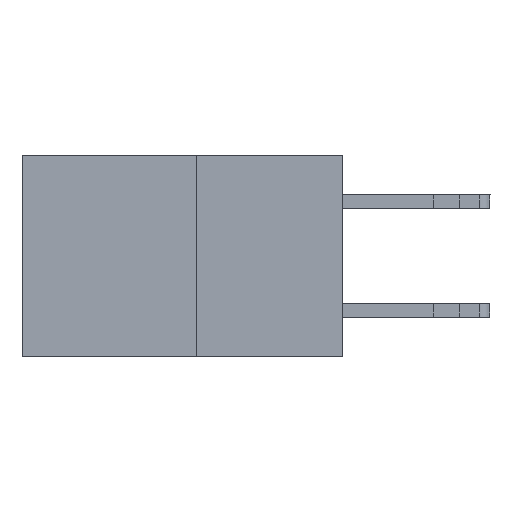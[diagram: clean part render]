
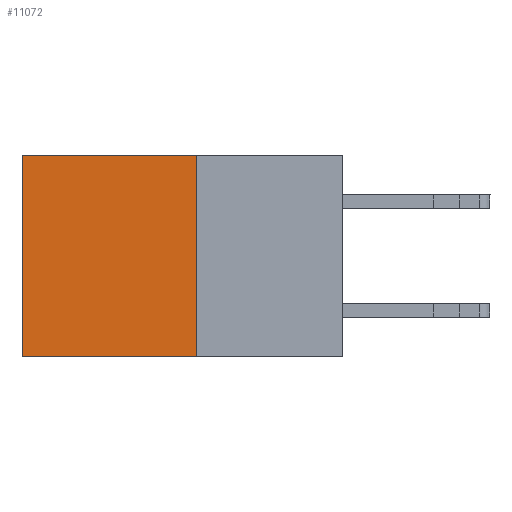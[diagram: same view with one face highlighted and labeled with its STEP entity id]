
A CAD part, left-side view. The second image highlights one B-rep face of the part: STEP entity #11072.
In plain terms, the highlighted planar face has unit normal (-1, 0, 0).
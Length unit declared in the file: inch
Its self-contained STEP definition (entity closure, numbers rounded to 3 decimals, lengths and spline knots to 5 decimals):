
#568 = EDGE_LOOP ( 'NONE', ( #12372, #11966, #10330, #10537 ) ) ;
#2612 = FACE_OUTER_BOUND ( 'NONE', #568, .T. ) ;
#2632 = CARTESIAN_POINT ( 'NONE',  ( 0.277, 0.27, -0.37 ) ) ;
#2668 = CARTESIAN_POINT ( 'NONE',  ( 0.277, 0.59, 0. ) ) ;
#2954 = VECTOR ( 'NONE', #13649, 39.37008 ) ;
#3480 = VECTOR ( 'NONE', #8361, 39.37008 ) ;
#4029 = DIRECTION ( 'NONE',  ( 0., 0., -1. ) ) ;
#4634 = EDGE_CURVE ( 'NONE', #5257, #15566, #16468, .T. ) ;
#4862 = CARTESIAN_POINT ( 'NONE',  ( 0.277, 0.27, 0. ) ) ;
#5257 = VERTEX_POINT ( 'NONE', #14742 ) ;
#6990 = CARTESIAN_POINT ( 'NONE',  ( 0.277, 0.27, -0.37 ) ) ;
#7020 = LINE ( 'NONE', #7182, #3480 ) ;
#7182 = CARTESIAN_POINT ( 'NONE',  ( 0.277, 0.59, -0.37 ) ) ;
#7238 = CARTESIAN_POINT ( 'NONE',  ( 0.277, 0.59, -0.37 ) ) ;
#8361 = DIRECTION ( 'NONE',  ( 0., 0., -1. ) ) ;
#8503 = LINE ( 'NONE', #6990, #2954 ) ;
#10330 = ORIENTED_EDGE ( 'NONE', *, *, #10469, .F. ) ;
#10469 = EDGE_CURVE ( 'NONE', #5257, #13905, #11695, .T. ) ;
#10500 = PLANE ( 'NONE',  #13161 ) ;
#10537 = ORIENTED_EDGE ( 'NONE', *, *, #4634, .T. ) ;
#10772 = VECTOR ( 'NONE', #15183, 39.37008 ) ;
#11072 = ADVANCED_FACE ( 'NONE', ( #2612 ), #10500, .F. ) ;
#11477 = CARTESIAN_POINT ( 'NONE',  ( 0.277, 0.27, -0.37 ) ) ;
#11613 = DIRECTION ( 'NONE',  ( 0., 0., -1. ) ) ;
#11695 = LINE ( 'NONE', #2632, #12873 ) ;
#11966 = ORIENTED_EDGE ( 'NONE', *, *, #14283, .F. ) ;
#12372 = ORIENTED_EDGE ( 'NONE', *, *, #15162, .T. ) ;
#12873 = VECTOR ( 'NONE', #11613, 39.37008 ) ;
#13161 = AXIS2_PLACEMENT_3D ( 'NONE', #15636, #16669, #4029 ) ;
#13649 = DIRECTION ( 'NONE',  ( 0., 1., 0. ) ) ;
#13905 = VERTEX_POINT ( 'NONE', #11477 ) ;
#14249 = VERTEX_POINT ( 'NONE', #7238 ) ;
#14283 = EDGE_CURVE ( 'NONE', #13905, #14249, #8503, .T. ) ;
#14742 = CARTESIAN_POINT ( 'NONE',  ( 0.277, 0.27, 0. ) ) ;
#15162 = EDGE_CURVE ( 'NONE', #15566, #14249, #7020, .T. ) ;
#15183 = DIRECTION ( 'NONE',  ( 0., 1., 0. ) ) ;
#15566 = VERTEX_POINT ( 'NONE', #2668 ) ;
#15636 = CARTESIAN_POINT ( 'NONE',  ( 0.277, 0.27, -0.37 ) ) ;
#16468 = LINE ( 'NONE', #4862, #10772 ) ;
#16669 = DIRECTION ( 'NONE',  ( 1., 0., 0. ) ) ;
